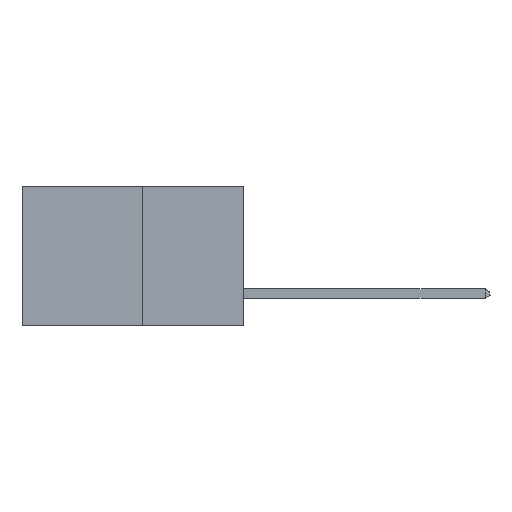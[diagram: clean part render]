
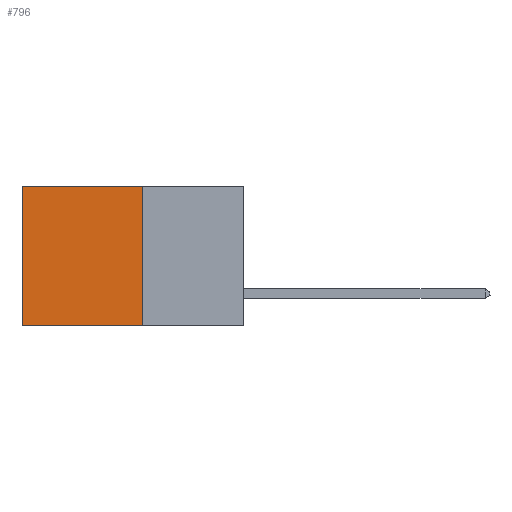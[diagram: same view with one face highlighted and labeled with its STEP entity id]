
A CAD part, left-side view. The second image highlights one B-rep face of the part: STEP entity #796.
In plain terms, the highlighted planar face has unit normal (-1, 0, 0).
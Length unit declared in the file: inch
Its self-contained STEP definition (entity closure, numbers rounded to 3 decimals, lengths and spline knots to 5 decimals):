
#267 = CARTESIAN_POINT ( 'NONE',  ( 0.277, 0.27, -0.37 ) ) ;
#416 = ORIENTED_EDGE ( 'NONE', *, *, #5159, .T. ) ;
#446 = CARTESIAN_POINT ( 'NONE',  ( 0.277, 0.27, 0. ) ) ;
#521 = VECTOR ( 'NONE', #4056, 39.37008 ) ;
#568 = ORIENTED_EDGE ( 'NONE', *, *, #8595, .F. ) ;
#796 = ADVANCED_FACE ( 'NONE', ( #9013 ), #2362, .F. ) ;
#891 = VERTEX_POINT ( 'NONE', #898 ) ;
#898 = CARTESIAN_POINT ( 'NONE',  ( 0.277, 0.27, -0.37 ) ) ;
#1043 = LINE ( 'NONE', #267, #4657 ) ;
#1490 = EDGE_CURVE ( 'NONE', #2255, #5936, #6130, .T. ) ;
#2114 = AXIS2_PLACEMENT_3D ( 'NONE', #4101, #4238, #2415 ) ;
#2255 = VERTEX_POINT ( 'NONE', #2696 ) ;
#2362 = PLANE ( 'NONE',  #2114 ) ;
#2415 = DIRECTION ( 'NONE',  ( 0., 0., -1. ) ) ;
#2542 = ORIENTED_EDGE ( 'NONE', *, *, #8579, .F. ) ;
#2631 = VECTOR ( 'NONE', #8671, 39.37008 ) ;
#2696 = CARTESIAN_POINT ( 'NONE',  ( 0.277, 0.59, 0. ) ) ;
#3181 = DIRECTION ( 'NONE',  ( 0., 0., -1. ) ) ;
#3207 = DIRECTION ( 'NONE',  ( 0., 1., 0. ) ) ;
#3900 = EDGE_LOOP ( 'NONE', ( #6809, #568, #2542, #416 ) ) ;
#4056 = DIRECTION ( 'NONE',  ( 0., 1., 0. ) ) ;
#4101 = CARTESIAN_POINT ( 'NONE',  ( 0.277, 0.27, -0.37 ) ) ;
#4238 = DIRECTION ( 'NONE',  ( 1., 0., 0. ) ) ;
#4657 = VECTOR ( 'NONE', #3207, 39.37008 ) ;
#4865 = VECTOR ( 'NONE', #3181, 39.37008 ) ;
#5159 = EDGE_CURVE ( 'NONE', #5217, #2255, #6221, .T. ) ;
#5217 = VERTEX_POINT ( 'NONE', #8342 ) ;
#5270 = CARTESIAN_POINT ( 'NONE',  ( 0.277, 0.27, -0.37 ) ) ;
#5936 = VERTEX_POINT ( 'NONE', #9068 ) ;
#6130 = LINE ( 'NONE', #8777, #2631 ) ;
#6221 = LINE ( 'NONE', #446, #521 ) ;
#6719 = LINE ( 'NONE', #5270, #4865 ) ;
#6809 = ORIENTED_EDGE ( 'NONE', *, *, #1490, .T. ) ;
#8342 = CARTESIAN_POINT ( 'NONE',  ( 0.277, 0.27, 0. ) ) ;
#8579 = EDGE_CURVE ( 'NONE', #5217, #891, #6719, .T. ) ;
#8595 = EDGE_CURVE ( 'NONE', #891, #5936, #1043, .T. ) ;
#8671 = DIRECTION ( 'NONE',  ( 0., 0., -1. ) ) ;
#8777 = CARTESIAN_POINT ( 'NONE',  ( 0.277, 0.59, -0.37 ) ) ;
#9013 = FACE_OUTER_BOUND ( 'NONE', #3900, .T. ) ;
#9068 = CARTESIAN_POINT ( 'NONE',  ( 0.277, 0.59, -0.37 ) ) ;
